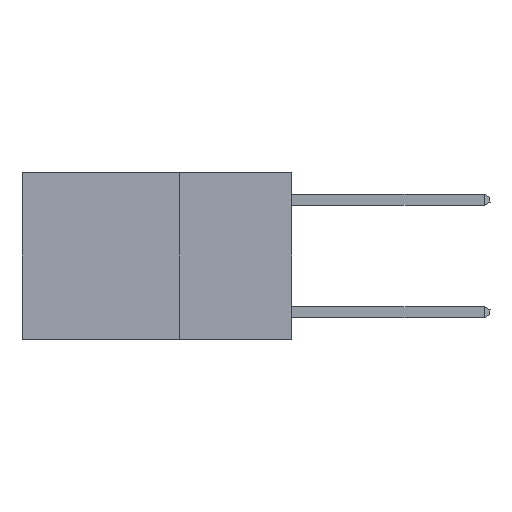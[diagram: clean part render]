
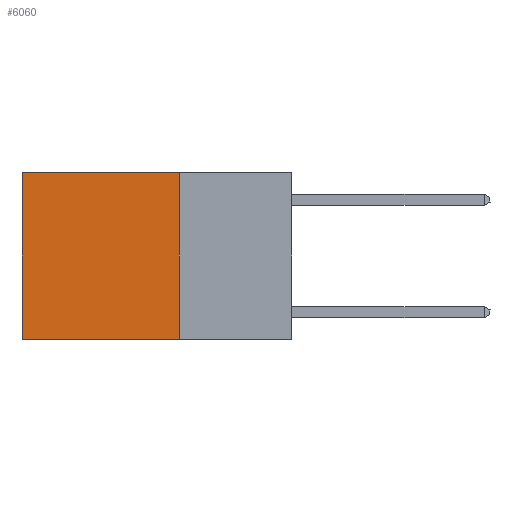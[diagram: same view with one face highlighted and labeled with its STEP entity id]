
A CAD part, left-side view. The second image highlights one B-rep face of the part: STEP entity #6060.
In plain terms, the highlighted planar face has unit normal (-1, 0, 0).
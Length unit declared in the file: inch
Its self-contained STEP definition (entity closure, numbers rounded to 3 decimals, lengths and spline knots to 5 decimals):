
#97 = EDGE_CURVE ( 'NONE', #220, #7627, #9502, .T. ) ;
#112 = EDGE_CURVE ( 'NONE', #1669, #7627, #10501, .T. ) ;
#220 = VERTEX_POINT ( 'NONE', #7957 ) ;
#727 = DIRECTION ( 'NONE',  ( 0., 1., 0. ) ) ;
#776 = DIRECTION ( 'NONE',  ( 0., 1., 0. ) ) ;
#1033 = CARTESIAN_POINT ( 'NONE',  ( 0.2625, 0.25, 0. ) ) ;
#1669 = VERTEX_POINT ( 'NONE', #5251 ) ;
#1699 = CARTESIAN_POINT ( 'NONE',  ( 0.2625, 0.25, 0. ) ) ;
#1935 = DIRECTION ( 'NONE',  ( 0., 0., -1. ) ) ;
#2135 = LINE ( 'NONE', #4668, #8865 ) ;
#2391 = CARTESIAN_POINT ( 'NONE',  ( 0.2625, 0.6, -0.37 ) ) ;
#2573 = CARTESIAN_POINT ( 'NONE',  ( 0.2625, 0.6, 0. ) ) ;
#2784 = LINE ( 'NONE', #1699, #4304 ) ;
#2882 = DIRECTION ( 'NONE',  ( 0., 0., -1. ) ) ;
#3246 = CARTESIAN_POINT ( 'NONE',  ( 0.2625, 0.25, -0.37 ) ) ;
#4304 = VECTOR ( 'NONE', #776, 39.37008 ) ;
#4564 = EDGE_CURVE ( 'NONE', #5683, #1669, #2784, .T. ) ;
#4584 = DIRECTION ( 'NONE',  ( 0., 0., -1. ) ) ;
#4668 = CARTESIAN_POINT ( 'NONE',  ( 0.2625, 0.25, 0. ) ) ;
#4669 = ORIENTED_EDGE ( 'NONE', *, *, #112, .T. ) ;
#4983 = VECTOR ( 'NONE', #1935, 39.37008 ) ;
#5251 = CARTESIAN_POINT ( 'NONE',  ( 0.2625, 0.6, 0. ) ) ;
#5683 = VERTEX_POINT ( 'NONE', #10712 ) ;
#6060 = ADVANCED_FACE ( 'NONE', ( #8318 ), #11743, .F. ) ;
#6422 = ORIENTED_EDGE ( 'NONE', *, *, #97, .F. ) ;
#7379 = EDGE_CURVE ( 'NONE', #5683, #220, #2135, .T. ) ;
#7627 = VERTEX_POINT ( 'NONE', #2391 ) ;
#7957 = CARTESIAN_POINT ( 'NONE',  ( 0.2625, 0.25, -0.37 ) ) ;
#8318 = FACE_OUTER_BOUND ( 'NONE', #8322, .T. ) ;
#8322 = EDGE_LOOP ( 'NONE', ( #4669, #6422, #10861, #11045 ) ) ;
#8865 = VECTOR ( 'NONE', #2882, 39.37008 ) ;
#9502 = LINE ( 'NONE', #3246, #11388 ) ;
#10079 = AXIS2_PLACEMENT_3D ( 'NONE', #1033, #10128, #4584 ) ;
#10128 = DIRECTION ( 'NONE',  ( 1., 0., 0. ) ) ;
#10501 = LINE ( 'NONE', #2573, #4983 ) ;
#10712 = CARTESIAN_POINT ( 'NONE',  ( 0.2625, 0.25, 0. ) ) ;
#10861 = ORIENTED_EDGE ( 'NONE', *, *, #7379, .F. ) ;
#11045 = ORIENTED_EDGE ( 'NONE', *, *, #4564, .T. ) ;
#11388 = VECTOR ( 'NONE', #727, 39.37008 ) ;
#11743 = PLANE ( 'NONE',  #10079 ) ;
